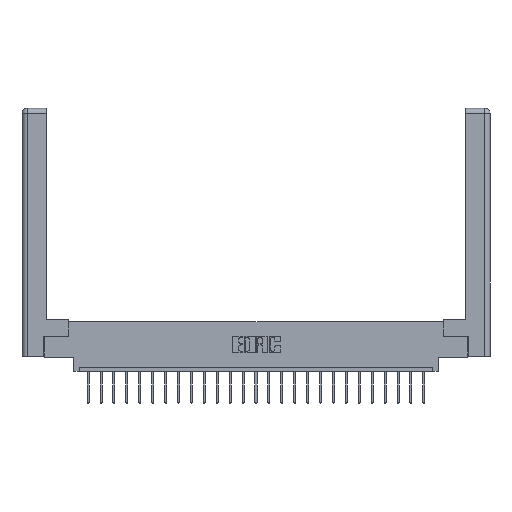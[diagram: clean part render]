
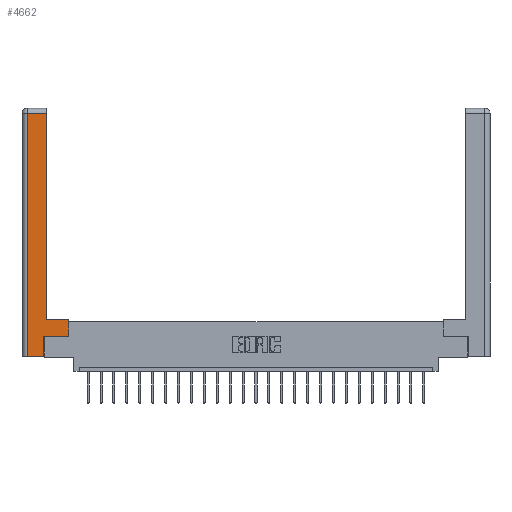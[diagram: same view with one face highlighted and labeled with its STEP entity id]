
A CAD part, top view. The second image highlights one B-rep face of the part: STEP entity #4662.
In plain terms, the highlighted planar face has unit normal (0, 0, 1).
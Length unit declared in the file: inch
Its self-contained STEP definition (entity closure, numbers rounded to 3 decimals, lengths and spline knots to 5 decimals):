
#325 = VECTOR ( 'NONE', #11206, 39.37008 ) ;
#381 = EDGE_CURVE ( 'NONE', #7160, #11091, #17361, .T. ) ;
#1089 = VECTOR ( 'NONE', #16678, 39.37008 ) ;
#1259 = ORIENTED_EDGE ( 'NONE', *, *, #2286, .T. ) ;
#2235 = EDGE_CURVE ( 'NONE', #12262, #9907, #13353, .T. ) ;
#2286 = EDGE_CURVE ( 'NONE', #3058, #18410, #3175, .T. ) ;
#2706 = CARTESIAN_POINT ( 'NONE',  ( 0.0615, 0., 0. ) ) ;
#3058 = VERTEX_POINT ( 'NONE', #21264 ) ;
#3175 = LINE ( 'NONE', #5295, #1089 ) ;
#3843 = CARTESIAN_POINT ( 'NONE',  ( 0.0615, 2.94, 0. ) ) ;
#4662 = ADVANCED_FACE ( 'NONE', ( #12968 ), #5081, .F. ) ;
#5081 = PLANE ( 'NONE',  #9290 ) ;
#5295 = CARTESIAN_POINT ( 'NONE',  ( 0.565, 0.45, 0. ) ) ;
#5568 = VERTEX_POINT ( 'NONE', #21014 ) ;
#6485 = CARTESIAN_POINT ( 'NONE',  ( 0.0615, 2.94, 0. ) ) ;
#7160 = VERTEX_POINT ( 'NONE', #14295 ) ;
#7719 = CARTESIAN_POINT ( 'NONE',  ( 0.295, 3., 0. ) ) ;
#7989 = DIRECTION ( 'NONE',  ( -1., 0., 0. ) ) ;
#8068 = ORIENTED_EDGE ( 'NONE', *, *, #381, .T. ) ;
#8786 = VECTOR ( 'NONE', #11532, 39.37008 ) ;
#9143 = VECTOR ( 'NONE', #21434, 39.37008 ) ;
#9270 = EDGE_CURVE ( 'NONE', #12702, #3058, #10411, .T. ) ;
#9290 = AXIS2_PLACEMENT_3D ( 'NONE', #16631, #18537, #16306 ) ;
#9907 = VERTEX_POINT ( 'NONE', #10133 ) ;
#10133 = CARTESIAN_POINT ( 'NONE',  ( 0.0615, 0., 0. ) ) ;
#10411 = LINE ( 'NONE', #22976, #13391 ) ;
#11091 = VERTEX_POINT ( 'NONE', #11597 ) ;
#11206 = DIRECTION ( 'NONE',  ( 1., 0., 0. ) ) ;
#11532 = DIRECTION ( 'NONE',  ( -1., 0., 0. ) ) ;
#11597 = CARTESIAN_POINT ( 'NONE',  ( 0.295, 2.94, 0. ) ) ;
#12116 = ORIENTED_EDGE ( 'NONE', *, *, #22259, .T. ) ;
#12262 = VERTEX_POINT ( 'NONE', #6485 ) ;
#12581 = EDGE_CURVE ( 'NONE', #5568, #12702, #23804, .T. ) ;
#12702 = VERTEX_POINT ( 'NONE', #20245 ) ;
#12968 = FACE_OUTER_BOUND ( 'NONE', #14796, .T. ) ;
#13353 = LINE ( 'NONE', #2706, #16378 ) ;
#13376 = CARTESIAN_POINT ( 'NONE',  ( 0.265, 0., 0. ) ) ;
#13391 = VECTOR ( 'NONE', #15292, 39.37008 ) ;
#13539 = VECTOR ( 'NONE', #7989, 39.37008 ) ;
#13697 = EDGE_CURVE ( 'NONE', #18410, #7160, #18040, .T. ) ;
#14295 = CARTESIAN_POINT ( 'NONE',  ( 0.295, 0.45, 0. ) ) ;
#14457 = EDGE_CURVE ( 'NONE', #9907, #5568, #15320, .T. ) ;
#14796 = EDGE_LOOP ( 'NONE', ( #8068, #12116, #22271, #22800, #24030, #22990, #1259, #16519 ) ) ;
#15292 = DIRECTION ( 'NONE',  ( 1., 0., 0. ) ) ;
#15320 = LINE ( 'NONE', #13376, #325 ) ;
#16306 = DIRECTION ( 'NONE',  ( -1., 0., 0. ) ) ;
#16378 = VECTOR ( 'NONE', #21942, 39.37008 ) ;
#16519 = ORIENTED_EDGE ( 'NONE', *, *, #13697, .T. ) ;
#16631 = CARTESIAN_POINT ( 'NONE',  ( 0., 0., 0. ) ) ;
#16678 = DIRECTION ( 'NONE',  ( 0., 1., 0. ) ) ;
#17361 = LINE ( 'NONE', #7719, #20927 ) ;
#18040 = LINE ( 'NONE', #21625, #13539 ) ;
#18410 = VERTEX_POINT ( 'NONE', #21457 ) ;
#18537 = DIRECTION ( 'NONE',  ( 0., 0., -1. ) ) ;
#19345 = CARTESIAN_POINT ( 'NONE',  ( 0.265, 0.245, 0. ) ) ;
#20245 = CARTESIAN_POINT ( 'NONE',  ( 0.265, 0.245, 0. ) ) ;
#20927 = VECTOR ( 'NONE', #22950, 39.37008 ) ;
#21014 = CARTESIAN_POINT ( 'NONE',  ( 0.265, 0., 0. ) ) ;
#21264 = CARTESIAN_POINT ( 'NONE',  ( 0.565, 0.245, 0. ) ) ;
#21434 = DIRECTION ( 'NONE',  ( 0., 1., 0. ) ) ;
#21457 = CARTESIAN_POINT ( 'NONE',  ( 0.565, 0.45, 0. ) ) ;
#21625 = CARTESIAN_POINT ( 'NONE',  ( 0.295, 0.45, 0. ) ) ;
#21942 = DIRECTION ( 'NONE',  ( 0., -1., 0. ) ) ;
#22259 = EDGE_CURVE ( 'NONE', #11091, #12262, #24037, .T. ) ;
#22271 = ORIENTED_EDGE ( 'NONE', *, *, #2235, .T. ) ;
#22800 = ORIENTED_EDGE ( 'NONE', *, *, #14457, .T. ) ;
#22950 = DIRECTION ( 'NONE',  ( 0., 1., 0. ) ) ;
#22976 = CARTESIAN_POINT ( 'NONE',  ( 0.565, 0.245, 0. ) ) ;
#22990 = ORIENTED_EDGE ( 'NONE', *, *, #9270, .T. ) ;
#23804 = LINE ( 'NONE', #19345, #9143 ) ;
#24030 = ORIENTED_EDGE ( 'NONE', *, *, #12581, .T. ) ;
#24037 = LINE ( 'NONE', #3843, #8786 ) ;
